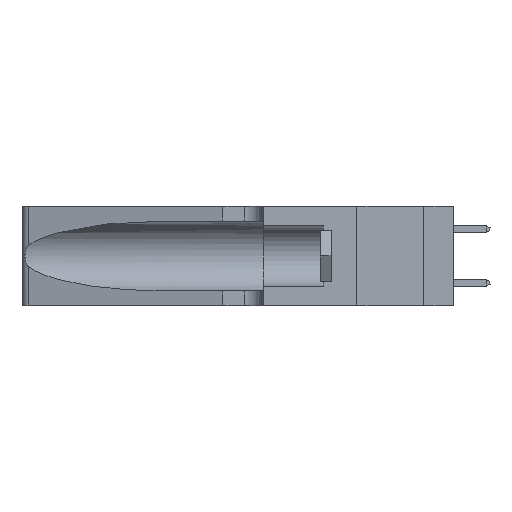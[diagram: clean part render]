
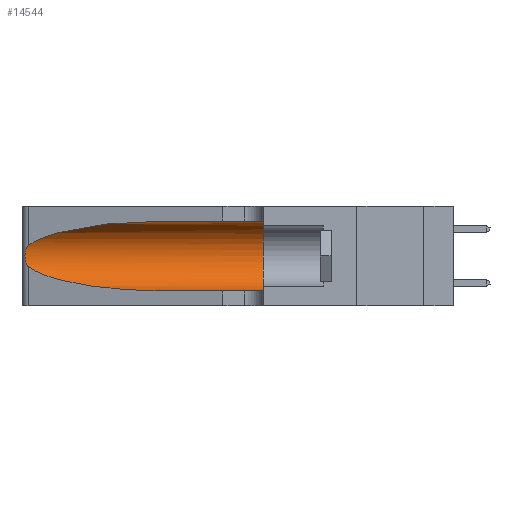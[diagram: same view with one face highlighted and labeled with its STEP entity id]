
A CAD part, left-side view. The second image highlights one B-rep face of the part: STEP entity #14544.
In plain terms, the highlighted cylindrical face has radius 3.308 mm (diameter 6.617 mm), a partial arc.
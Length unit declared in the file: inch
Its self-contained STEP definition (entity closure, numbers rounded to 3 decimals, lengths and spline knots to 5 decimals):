
#688 = EDGE_CURVE ( 'NONE', #2858, #11287, #14615, .T. ) ;
#699 = EDGE_CURVE ( 'NONE', #8801, #7247, #8140, .T. ) ;
#867 = CARTESIAN_POINT ( 'NONE',  ( 0.1305, 0.72297, 0.05475 ) ) ;
#2389 = CARTESIAN_POINT ( 'NONE',  ( 0.25487, 1.22718, 0.14631 ) ) ;
#2554 = LINE ( 'NONE', #5905, #18746 ) ;
#2694 = CARTESIAN_POINT ( 'NONE',  ( 0.1305, 0.72297, 0.31525 ) ) ;
#2707 = ORIENTED_EDGE ( 'NONE', *, *, #699, .T. ) ;
#2858 = VERTEX_POINT ( 'NONE', #14403 ) ;
#3231 = LINE ( 'NONE', #14371, #15251 ) ;
#4201 =( BOUNDED_CURVE ( )  B_SPLINE_CURVE ( 3, ( #17568, #8198, #19133, #9775 ),
 .UNSPECIFIED., .F., .F. ) 
 B_SPLINE_CURVE_WITH_KNOTS ( ( 4, 4 ),
 ( 1.5708, 2.84003 ),
 .UNSPECIFIED. ) 
 CURVE ( )  GEOMETRIC_REPRESENTATION_ITEM ( )  RATIONAL_B_SPLINE_CURVE ( ( 1., 0.87, 0.87, 1. ) ) 
 REPRESENTATION_ITEM ( '' )  );
#5544 = CARTESIAN_POINT ( 'NONE',  ( 0.2373, 1.15595, 0.08982 ) ) ;
#5552 = AXIS2_PLACEMENT_3D ( 'NONE', #12535, #15990, #16391 ) ;
#5628 =( BOUNDED_CURVE ( )  B_SPLINE_CURVE ( 3, ( #2389, #5544, #10319, #867 ),
 .UNSPECIFIED., .F., .F. ) 
 B_SPLINE_CURVE_WITH_KNOTS ( ( 4, 4 ),
 ( 3.44316, 4.71239 ),
 .UNSPECIFIED. ) 
 CURVE ( )  GEOMETRIC_REPRESENTATION_ITEM ( )  RATIONAL_B_SPLINE_CURVE ( ( 1., 0.87, 0.87, 1. ) ) 
 REPRESENTATION_ITEM ( '' )  );
#5905 = CARTESIAN_POINT ( 'NONE',  ( 0.1305, 1.61858, 0.31525 ) ) ;
#6178 = AXIS2_PLACEMENT_3D ( 'NONE', #16456, #7086, #18034 ) ;
#6263 = CARTESIAN_POINT ( 'NONE',  ( 0.25487, 1.22718, 0.22369 ) ) ;
#6322 = ORIENTED_EDGE ( 'NONE', *, *, #15572, .T. ) ;
#6691 = CARTESIAN_POINT ( 'NONE',  ( 0.26018, 1.23835, 0.19895 ) ) ;
#6818 = CARTESIAN_POINT ( 'NONE',  ( 0.26075, 1.23896, 0.19203 ) ) ;
#7086 = DIRECTION ( 'NONE',  ( 0., -1., 0. ) ) ;
#7247 = VERTEX_POINT ( 'NONE', #10628 ) ;
#7498 = DIRECTION ( 'NONE',  ( 0., -1., 0. ) ) ;
#7771 = CARTESIAN_POINT ( 'NONE',  ( 0.1305, 0.72297, 0.05475 ) ) ;
#8015 = ORIENTED_EDGE ( 'NONE', *, *, #14050, .F. ) ;
#8140 = B_SPLINE_CURVE_WITH_KNOTS ( 'NONE', 3,
 ( #11356, #10464, #16037, #19538, #14646, #6691, #6818, #10801, #16547, #16116, #16191, #10932, #18662, #16012 ),
 .UNSPECIFIED., .F., .F.,
 ( 4, 2, 2, 2, 2, 2, 4 ),
 ( 0., 0.00027, 0.00053, 0.00107, 0.0016, 0.00187, 0.00214 ),
 .UNSPECIFIED. ) ;
#8198 = CARTESIAN_POINT ( 'NONE',  ( 0.18966, 0.96281, 0.31525 ) ) ;
#8616 = VERTEX_POINT ( 'NONE', #2694 ) ;
#8801 = VERTEX_POINT ( 'NONE', #6263 ) ;
#9316 = VERTEX_POINT ( 'NONE', #7771 ) ;
#9775 = CARTESIAN_POINT ( 'NONE',  ( 0.25487, 1.22718, 0.22369 ) ) ;
#10319 = CARTESIAN_POINT ( 'NONE',  ( 0.18966, 0.96281, 0.05475 ) ) ;
#10464 = CARTESIAN_POINT ( 'NONE',  ( 0.25555, 1.22994, 0.2215 ) ) ;
#10628 = CARTESIAN_POINT ( 'NONE',  ( 0.25487, 1.22718, 0.14631 ) ) ;
#10632 = ORIENTED_EDGE ( 'NONE', *, *, #14589, .T. ) ;
#10676 = CARTESIAN_POINT ( 'NONE',  ( 0.1305, 0.35, 0.05475 ) ) ;
#10706 = EDGE_LOOP ( 'NONE', ( #11134, #2707, #10632, #6322, #12409, #8015 ) ) ;
#10801 = CARTESIAN_POINT ( 'NONE',  ( 0.26075, 1.23896, 0.178 ) ) ;
#10932 = CARTESIAN_POINT ( 'NONE',  ( 0.25639, 1.23186, 0.15144 ) ) ;
#11134 = ORIENTED_EDGE ( 'NONE', *, *, #16214, .T. ) ;
#11287 = VERTEX_POINT ( 'NONE', #10676 ) ;
#11356 = CARTESIAN_POINT ( 'NONE',  ( 0.25487, 1.22718, 0.22369 ) ) ;
#12409 = ORIENTED_EDGE ( 'NONE', *, *, #688, .F. ) ;
#12535 = CARTESIAN_POINT ( 'NONE',  ( 0.1305, 0.35, 0.185 ) ) ;
#12882 = DIRECTION ( 'NONE',  ( 0., -1., 0. ) ) ;
#14050 = EDGE_CURVE ( 'NONE', #8616, #2858, #2554, .T. ) ;
#14371 = CARTESIAN_POINT ( 'NONE',  ( 0.1305, 1.61858, 0.05475 ) ) ;
#14403 = CARTESIAN_POINT ( 'NONE',  ( 0.1305, 0.35, 0.31525 ) ) ;
#14544 = ADVANCED_FACE ( 'NONE', ( #17763 ), #17272, .F. ) ;
#14589 = EDGE_CURVE ( 'NONE', #7247, #9316, #5628, .T. ) ;
#14615 = CIRCLE ( 'NONE', #5552, 0.13025 ) ;
#14646 = CARTESIAN_POINT ( 'NONE',  ( 0.25854, 1.2359, 0.20912 ) ) ;
#15251 = VECTOR ( 'NONE', #12882, 39.37008 ) ;
#15572 = EDGE_CURVE ( 'NONE', #9316, #11287, #3231, .T. ) ;
#15990 = DIRECTION ( 'NONE',  ( 0., 1., 0. ) ) ;
#16012 = CARTESIAN_POINT ( 'NONE',  ( 0.25487, 1.22718, 0.14631 ) ) ;
#16037 = CARTESIAN_POINT ( 'NONE',  ( 0.25639, 1.23184, 0.21858 ) ) ;
#16116 = CARTESIAN_POINT ( 'NONE',  ( 0.25856, 1.23593, 0.16098 ) ) ;
#16191 = CARTESIAN_POINT ( 'NONE',  ( 0.25789, 1.23486, 0.15765 ) ) ;
#16214 = EDGE_CURVE ( 'NONE', #8616, #8801, #4201, .T. ) ;
#16391 = DIRECTION ( 'NONE',  ( 0., 0., 1. ) ) ;
#16456 = CARTESIAN_POINT ( 'NONE',  ( 0.1305, 1.61858, 0.185 ) ) ;
#16547 = CARTESIAN_POINT ( 'NONE',  ( 0.26017, 1.23833, 0.17102 ) ) ;
#17272 = CYLINDRICAL_SURFACE ( 'NONE', #6178, 0.13025 ) ;
#17568 = CARTESIAN_POINT ( 'NONE',  ( 0.1305, 0.72297, 0.31525 ) ) ;
#17763 = FACE_OUTER_BOUND ( 'NONE', #10706, .T. ) ;
#18034 = DIRECTION ( 'NONE',  ( 0., 0., -1. ) ) ;
#18662 = CARTESIAN_POINT ( 'NONE',  ( 0.25555, 1.22993, 0.14849 ) ) ;
#18746 = VECTOR ( 'NONE', #7498, 39.37008 ) ;
#19133 = CARTESIAN_POINT ( 'NONE',  ( 0.2373, 1.15595, 0.28018 ) ) ;
#19538 = CARTESIAN_POINT ( 'NONE',  ( 0.25787, 1.23484, 0.2124 ) ) ;
